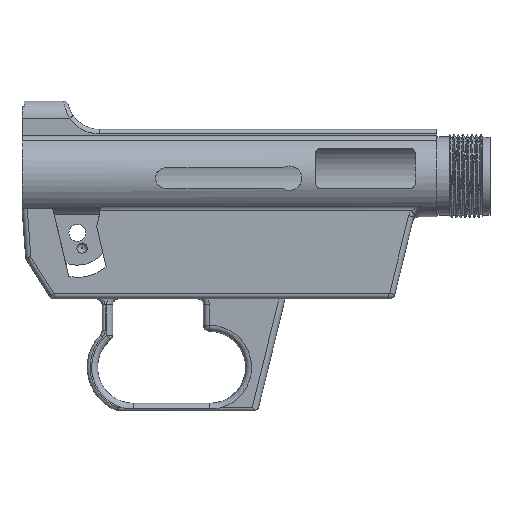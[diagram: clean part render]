
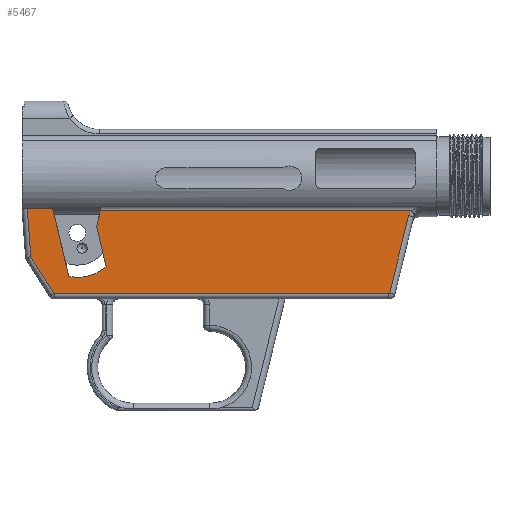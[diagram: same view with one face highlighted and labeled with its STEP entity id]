
A CAD part, left-side view. The second image highlights one B-rep face of the part: STEP entity #5467.
In plain terms, the highlighted planar face has unit normal (-1, 0, 0).
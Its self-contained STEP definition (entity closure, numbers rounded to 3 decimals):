
#123=B_SPLINE_CURVE_WITH_KNOTS('',3,(#8830,#8831,#8832,#8833),
 .UNSPECIFIED.,.F.,.F.,(4,4),(0.,0.178),.UNSPECIFIED.);
#283=PLANE('',#5918);
#483=FACE_OUTER_BOUND('',#790,.T.);
#790=EDGE_LOOP('',(#4102,#4103,#4104,#4105,#4106,#4107,#4108,#4109,#4110,
#4111,#4112,#4113,#4114,#4115));
#1183=LINE('',#8839,#1641);
#1184=LINE('',#8856,#1642);
#1186=LINE('',#8876,#1644);
#1188=LINE('',#8906,#1646);
#1191=LINE('',#8932,#1649);
#1192=LINE('',#8934,#1650);
#1193=LINE('',#8936,#1651);
#1194=LINE('',#8940,#1652);
#1195=LINE('',#8941,#1653);
#1641=VECTOR('',#6800,10.);
#1642=VECTOR('',#6811,10.);
#1644=VECTOR('',#6823,10.);
#1646=VECTOR('',#6833,10.);
#1649=VECTOR('',#6846,10.);
#1650=VECTOR('',#6847,10.);
#1651=VECTOR('',#6848,10.);
#1652=VECTOR('',#6851,10.);
#1653=VECTOR('',#6852,10.);
#2047=CIRCLE('',#5902,0.25);
#2051=CIRCLE('',#5907,0.25);
#2055=CIRCLE('',#5912,0.25);
#2058=CIRCLE('',#5919,14.884);
#2391=VERTEX_POINT('',#8793);
#2392=VERTEX_POINT('',#8823);
#2394=VERTEX_POINT('',#8835);
#2396=VERTEX_POINT('',#8849);
#2397=VERTEX_POINT('',#8854);
#2398=VERTEX_POINT('',#8866);
#2400=VERTEX_POINT('',#8872);
#2402=VERTEX_POINT('',#8886);
#2406=VERTEX_POINT('',#8905);
#2412=VERTEX_POINT('',#8931);
#2413=VERTEX_POINT('',#8933);
#2414=VERTEX_POINT('',#8935);
#2415=VERTEX_POINT('',#8937);
#2416=VERTEX_POINT('',#8939);
#3033=EDGE_CURVE('',#2391,#2392,#123,.T.);
#3036=EDGE_CURVE('',#2392,#2394,#1183,.T.);
#3039=EDGE_CURVE('',#2394,#2396,#2047,.T.);
#3041=EDGE_CURVE('',#2396,#2397,#1184,.T.);
#3044=EDGE_CURVE('',#2397,#2398,#2051,.T.);
#3047=EDGE_CURVE('',#2398,#2400,#1186,.T.);
#3050=EDGE_CURVE('',#2400,#2402,#2055,.T.);
#3053=EDGE_CURVE('',#2402,#2406,#1188,.T.);
#3061=EDGE_CURVE('',#2412,#2391,#1191,.T.);
#3062=EDGE_CURVE('',#2412,#2413,#1192,.T.);
#3063=EDGE_CURVE('',#2413,#2414,#1193,.T.);
#3064=EDGE_CURVE('',#2414,#2415,#2058,.T.);
#3065=EDGE_CURVE('',#2415,#2416,#1194,.T.);
#3066=EDGE_CURVE('',#2406,#2416,#1195,.T.);
#4102=ORIENTED_EDGE('',*,*,#3053,.F.);
#4103=ORIENTED_EDGE('',*,*,#3050,.F.);
#4104=ORIENTED_EDGE('',*,*,#3047,.F.);
#4105=ORIENTED_EDGE('',*,*,#3044,.F.);
#4106=ORIENTED_EDGE('',*,*,#3041,.F.);
#4107=ORIENTED_EDGE('',*,*,#3039,.F.);
#4108=ORIENTED_EDGE('',*,*,#3036,.F.);
#4109=ORIENTED_EDGE('',*,*,#3033,.F.);
#4110=ORIENTED_EDGE('',*,*,#3061,.F.);
#4111=ORIENTED_EDGE('',*,*,#3062,.T.);
#4112=ORIENTED_EDGE('',*,*,#3063,.T.);
#4113=ORIENTED_EDGE('',*,*,#3064,.T.);
#4114=ORIENTED_EDGE('',*,*,#3065,.T.);
#4115=ORIENTED_EDGE('',*,*,#3066,.F.);
#5467=ADVANCED_FACE('',(#483),#283,.T.);
#5902=AXIS2_PLACEMENT_3D('',#8852,#6805,#6806);
#5907=AXIS2_PLACEMENT_3D('',#8870,#6816,#6817);
#5912=AXIS2_PLACEMENT_3D('',#8890,#6828,#6829);
#5918=AXIS2_PLACEMENT_3D('',#8930,#6844,#6845);
#5919=AXIS2_PLACEMENT_3D('',#8938,#6849,#6850);
#6800=DIRECTION('',(0.,0.236,-0.972));
#6805=DIRECTION('center_axis',(1.,0.,0.));
#6806=DIRECTION('ref_axis',(0.,-0.618,-0.786));
#6811=DIRECTION('',(0.,1.,0.));
#6816=DIRECTION('center_axis',(1.,0.,0.));
#6817=DIRECTION('ref_axis',(0.,0.481,-0.877));
#6823=DIRECTION('',(0.,0.537,0.843));
#6828=DIRECTION('center_axis',(1.,0.,0.));
#6829=DIRECTION('ref_axis',(0.,0.949,-0.315));
#6833=DIRECTION('',(0.,0.073,0.997));
#6844=DIRECTION('center_axis',(-1.,0.,0.));
#6845=DIRECTION('ref_axis',(0.,0.,1.));
#6846=DIRECTION('',(0.,-1.,0.));
#6847=DIRECTION('',(0.,0.225,-0.974));
#6848=DIRECTION('',(0.,-0.225,-0.974));
#6849=DIRECTION('center_axis',(1.,0.,0.));
#6850=DIRECTION('ref_axis',(0.,-1.,0.));
#6851=DIRECTION('',(0.,0.229,0.973));
#6852=DIRECTION('',(0.,-1.,0.));
#8793=CARTESIAN_POINT('',(-8.475,-69.047,29.521));
#8823=CARTESIAN_POINT('',(-8.475,-68.314,27.907));
#8830=CARTESIAN_POINT('Ctrl Pts',(-8.475,-69.047,29.521));
#8831=CARTESIAN_POINT('Ctrl Pts',(-8.475,-68.705,29.035));
#8832=CARTESIAN_POINT('Ctrl Pts',(-8.475,-68.454,28.485));
#8833=CARTESIAN_POINT('Ctrl Pts',(-8.475,-68.314,27.907));
#8835=CARTESIAN_POINT('',(-8.475,-62.016,1.941));
#8839=CARTESIAN_POINT('',(-8.475,-59.885,-6.843));
#8849=CARTESIAN_POINT('',(-8.475,-61.773,1.75));
#8852=CARTESIAN_POINT('Origin',(-8.475,-61.773,2.));
#8854=CARTESIAN_POINT('',(-8.475,50.368,1.75));
#8856=CARTESIAN_POINT('',(-8.475,0.,1.75));
#8866=CARTESIAN_POINT('',(-8.475,50.579,1.866));
#8870=CARTESIAN_POINT('Origin',(-8.475,50.368,2.));
#8872=CARTESIAN_POINT('',(-8.475,58.313,14.01));
#8876=CARTESIAN_POINT('',(-8.475,46.861,-3.971));
#8886=CARTESIAN_POINT('',(-8.475,58.352,14.126));
#8890=CARTESIAN_POINT('Origin',(-8.475,58.102,14.145));
#8905=CARTESIAN_POINT('',(-8.475,59.549,30.45));
#8906=CARTESIAN_POINT('',(-8.475,58.284,13.198));
#8930=CARTESIAN_POINT('Origin',(-8.475,0.,0.));
#8931=CARTESIAN_POINT('',(-8.475,35.068,29.521));
#8932=CARTESIAN_POINT('',(-8.475,0.,29.521));
#8933=CARTESIAN_POINT('',(-8.475,36.258,24.36));
#8934=CARTESIAN_POINT('',(-8.475,37.307,19.808));
#8935=CARTESIAN_POINT('',(-8.475,33.128,10.797));
#8936=CARTESIAN_POINT('',(-8.475,32.672,8.823));
#8937=CARTESIAN_POINT('',(-8.475,45.62,7.575));
#8938=CARTESIAN_POINT('Origin',(-8.475,42.724,22.175));
#8939=CARTESIAN_POINT('',(-8.475,51.004,30.45));
#8940=CARTESIAN_POINT('',(-8.475,43.577,-1.101));
#8941=CARTESIAN_POINT('',(-8.475,61.304,30.45));
